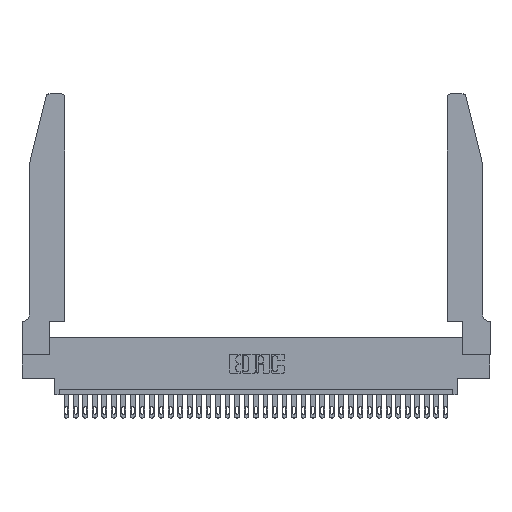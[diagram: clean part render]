
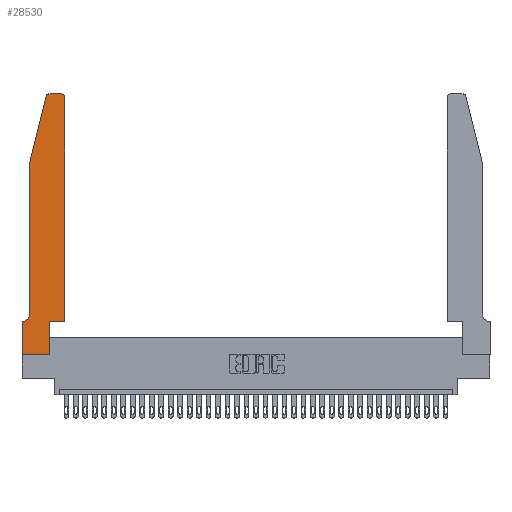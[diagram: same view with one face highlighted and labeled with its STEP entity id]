
A CAD part, top view. The second image highlights one B-rep face of the part: STEP entity #28530.
In plain terms, the highlighted planar face has unit normal (0, 0, 1).
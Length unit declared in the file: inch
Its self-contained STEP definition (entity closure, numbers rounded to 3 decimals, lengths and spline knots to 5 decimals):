
#89 = DIRECTION ( 'NONE',  ( 0., -1., 0. ) ) ;
#640 = VERTEX_POINT ( 'NONE', #14352 ) ;
#651 = VERTEX_POINT ( 'NONE', #11572 ) ;
#928 = EDGE_LOOP ( 'NONE', ( #27103, #12539, #35397, #7256, #33110, #13021, #27148, #5779, #35023, #6652, #22689, #16826 ) ) ;
#940 = EDGE_CURVE ( 'NONE', #19065, #27468, #12803, .T. ) ;
#1084 = EDGE_CURVE ( 'NONE', #10693, #6757, #2794, .T. ) ;
#1287 = VECTOR ( 'NONE', #28249, 39.37008 ) ;
#2507 = VERTEX_POINT ( 'NONE', #29769 ) ;
#2794 = LINE ( 'NONE', #20808, #10613 ) ;
#2865 = CARTESIAN_POINT ( 'NONE',  ( 0.2865, 0.35, 0.37 ) ) ;
#3385 = VERTEX_POINT ( 'NONE', #16463 ) ;
#3562 = CIRCLE ( 'NONE', #28659, 0.03 ) ;
#3672 = DIRECTION ( 'NONE',  ( 1., 0., 0. ) ) ;
#4352 = EDGE_CURVE ( 'NONE', #651, #640, #31106, .T. ) ;
#4444 = CARTESIAN_POINT ( 'NONE',  ( 0.4505, 0.35, 0.37 ) ) ;
#5180 = EDGE_CURVE ( 'NONE', #25121, #17767, #27589, .T. ) ;
#5278 = VECTOR ( 'NONE', #28088, 39.37008 ) ;
#5506 = CARTESIAN_POINT ( 'NONE',  ( 0.2865, 0., 0.37 ) ) ;
#5652 = VECTOR ( 'NONE', #17460, 39.37008 ) ;
#5779 = ORIENTED_EDGE ( 'NONE', *, *, #1084, .T. ) ;
#6652 = ORIENTED_EDGE ( 'NONE', *, *, #940, .T. ) ;
#6757 = VERTEX_POINT ( 'NONE', #5506 ) ;
#7256 = ORIENTED_EDGE ( 'NONE', *, *, #31247, .T. ) ;
#7278 = DIRECTION ( 'NONE',  ( 0., 0., 1. ) ) ;
#8921 = CARTESIAN_POINT ( 'NONE',  ( 0., 0., 0.37 ) ) ;
#9472 = EDGE_CURVE ( 'NONE', #6757, #19065, #20003, .T. ) ;
#9940 = LINE ( 'NONE', #8921, #1287 ) ;
#10613 = VECTOR ( 'NONE', #30282, 39.37008 ) ;
#10693 = VERTEX_POINT ( 'NONE', #28070 ) ;
#11196 = CARTESIAN_POINT ( 'NONE',  ( 0.0055, 0.42, 0.37 ) ) ;
#11572 = CARTESIAN_POINT ( 'NONE',  ( 0.4505, 2.72, 0.37 ) ) ;
#11935 = VERTEX_POINT ( 'NONE', #33932 ) ;
#12405 = EDGE_CURVE ( 'NONE', #2507, #10693, #9940, .T. ) ;
#12416 = DIRECTION ( 'NONE',  ( 0., 1., 0. ) ) ;
#12539 = ORIENTED_EDGE ( 'NONE', *, *, #33522, .T. ) ;
#12803 = LINE ( 'NONE', #29027, #24849 ) ;
#12832 = LINE ( 'NONE', #13871, #21514 ) ;
#12954 = EDGE_CURVE ( 'NONE', #3385, #11935, #31454, .T. ) ;
#13021 = ORIENTED_EDGE ( 'NONE', *, *, #35688, .T. ) ;
#13871 = CARTESIAN_POINT ( 'NONE',  ( 0.0755, 2., 0.37 ) ) ;
#14352 = CARTESIAN_POINT ( 'NONE',  ( 0.4205, 2.75, 0.37 ) ) ;
#14673 = CARTESIAN_POINT ( 'NONE',  ( 0.0055, 0.35, 0.37 ) ) ;
#16463 = CARTESIAN_POINT ( 'NONE',  ( 0.25487, 2.72718, 0.37 ) ) ;
#16695 = PLANE ( 'NONE',  #34757 ) ;
#16826 = ORIENTED_EDGE ( 'NONE', *, *, #4352, .T. ) ;
#16860 = DIRECTION ( 'NONE',  ( 0., 0., -1. ) ) ;
#16872 = CARTESIAN_POINT ( 'NONE',  ( 0.0755, 2., 0.37 ) ) ;
#17028 = DIRECTION ( 'NONE',  ( 1., 0., 0. ) ) ;
#17338 = CARTESIAN_POINT ( 'NONE',  ( 0.284, 2.75, 0.37 ) ) ;
#17460 = DIRECTION ( 'NONE',  ( -1., 0., 0. ) ) ;
#17480 = FACE_OUTER_BOUND ( 'NONE', #928, .T. ) ;
#17767 = VERTEX_POINT ( 'NONE', #14673 ) ;
#17796 = LINE ( 'NONE', #22901, #5652 ) ;
#18544 = LINE ( 'NONE', #4444, #25325 ) ;
#19065 = VERTEX_POINT ( 'NONE', #31610 ) ;
#19506 = CARTESIAN_POINT ( 'NONE',  ( 0., 0.35, 0.37 ) ) ;
#19703 = AXIS2_PLACEMENT_3D ( 'NONE', #33985, #33728, #3672 ) ;
#20003 = LINE ( 'NONE', #2865, #5278 ) ;
#20403 = VERTEX_POINT ( 'NONE', #17338 ) ;
#20808 = CARTESIAN_POINT ( 'NONE',  ( 0., 0., 0.37 ) ) ;
#21178 = VECTOR ( 'NONE', #25182, 39.37008 ) ;
#21296 = EDGE_CURVE ( 'NONE', #640, #20403, #17796, .T. ) ;
#21514 = VECTOR ( 'NONE', #89, 39.37008 ) ;
#21564 = CARTESIAN_POINT ( 'NONE',  ( 0.4505, 0.35, 0.37 ) ) ;
#21889 = CARTESIAN_POINT ( 'NONE',  ( 0.0755, 0.35, 0.37 ) ) ;
#22689 = ORIENTED_EDGE ( 'NONE', *, *, #26793, .T. ) ;
#22860 = VECTOR ( 'NONE', #35182, 39.37008 ) ;
#22901 = CARTESIAN_POINT ( 'NONE',  ( 0.2605, 2.75, 0.37 ) ) ;
#23854 = CARTESIAN_POINT ( 'NONE',  ( 0.284, 2.72, 0.37 ) ) ;
#24849 = VECTOR ( 'NONE', #31809, 39.37008 ) ;
#25002 = AXIS2_PLACEMENT_3D ( 'NONE', #11196, #16860, #33492 ) ;
#25121 = VERTEX_POINT ( 'NONE', #29454 ) ;
#25182 = DIRECTION ( 'NONE',  ( -0.239, -0.971, 0. ) ) ;
#25325 = VECTOR ( 'NONE', #12416, 39.37008 ) ;
#26793 = EDGE_CURVE ( 'NONE', #27468, #651, #18544, .T. ) ;
#27103 = ORIENTED_EDGE ( 'NONE', *, *, #21296, .T. ) ;
#27148 = ORIENTED_EDGE ( 'NONE', *, *, #12405, .T. ) ;
#27468 = VERTEX_POINT ( 'NONE', #21564 ) ;
#27589 = CIRCLE ( 'NONE', #25002, 0.07 ) ;
#28070 = CARTESIAN_POINT ( 'NONE',  ( 0., 0., 0.37 ) ) ;
#28088 = DIRECTION ( 'NONE',  ( 0., 1., 0. ) ) ;
#28249 = DIRECTION ( 'NONE',  ( 0., -1., 0. ) ) ;
#28530 = ADVANCED_FACE ( 'NONE', ( #17480 ), #16695, .T. ) ;
#28659 = AXIS2_PLACEMENT_3D ( 'NONE', #23854, #7278, #29346 ) ;
#29027 = CARTESIAN_POINT ( 'NONE',  ( 0.4505, 0.35, 0.37 ) ) ;
#29346 = DIRECTION ( 'NONE',  ( 1., 0., 0. ) ) ;
#29454 = CARTESIAN_POINT ( 'NONE',  ( 0.0755, 0.42, 0.37 ) ) ;
#29769 = CARTESIAN_POINT ( 'NONE',  ( 0., 0.35, 0.37 ) ) ;
#30173 = LINE ( 'NONE', #21889, #22860 ) ;
#30282 = DIRECTION ( 'NONE',  ( 1., 0., 0. ) ) ;
#30636 = DIRECTION ( 'NONE',  ( 0., 0., 1. ) ) ;
#31106 = CIRCLE ( 'NONE', #19703, 0.03 ) ;
#31247 = EDGE_CURVE ( 'NONE', #11935, #25121, #12832, .T. ) ;
#31454 = LINE ( 'NONE', #16872, #21178 ) ;
#31610 = CARTESIAN_POINT ( 'NONE',  ( 0.2865, 0.35, 0.37 ) ) ;
#31809 = DIRECTION ( 'NONE',  ( 1., 0., 0. ) ) ;
#33110 = ORIENTED_EDGE ( 'NONE', *, *, #5180, .T. ) ;
#33492 = DIRECTION ( 'NONE',  ( -1., 0., 0. ) ) ;
#33522 = EDGE_CURVE ( 'NONE', #20403, #3385, #3562, .T. ) ;
#33728 = DIRECTION ( 'NONE',  ( 0., 0., 1. ) ) ;
#33932 = CARTESIAN_POINT ( 'NONE',  ( 0.0755, 2., 0.37 ) ) ;
#33985 = CARTESIAN_POINT ( 'NONE',  ( 0.4205, 2.72, 0.37 ) ) ;
#34757 = AXIS2_PLACEMENT_3D ( 'NONE', #19506, #30636, #17028 ) ;
#35023 = ORIENTED_EDGE ( 'NONE', *, *, #9472, .T. ) ;
#35182 = DIRECTION ( 'NONE',  ( -1., 0., 0. ) ) ;
#35397 = ORIENTED_EDGE ( 'NONE', *, *, #12954, .T. ) ;
#35688 = EDGE_CURVE ( 'NONE', #17767, #2507, #30173, .T. ) ;
